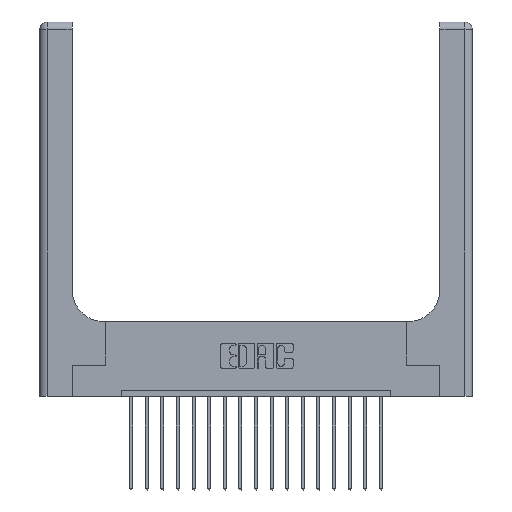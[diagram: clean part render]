
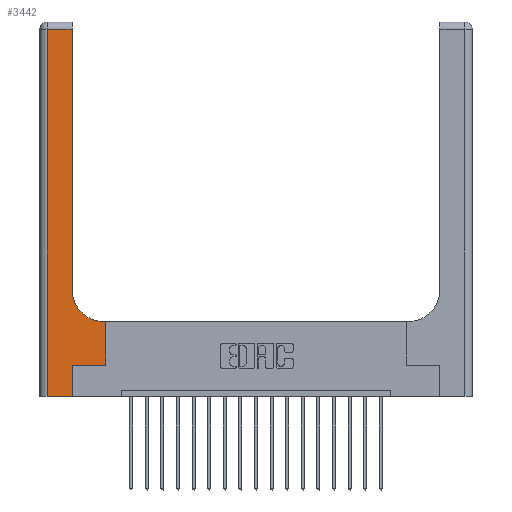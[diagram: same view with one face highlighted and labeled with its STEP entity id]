
A CAD part, top view. The second image highlights one B-rep face of the part: STEP entity #3442.
In plain terms, the highlighted planar face has unit normal (0, 0, 1).
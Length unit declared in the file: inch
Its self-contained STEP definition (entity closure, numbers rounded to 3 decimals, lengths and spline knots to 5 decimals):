
#392 = EDGE_CURVE ( 'NONE', #11306, #8371, #546, .T. ) ;
#546 = LINE ( 'NONE', #15489, #1305 ) ;
#905 = ORIENTED_EDGE ( 'NONE', *, *, #8305, .T. ) ;
#1125 = CARTESIAN_POINT ( 'NONE',  ( 0.528, 0.6, 0.37 ) ) ;
#1305 = VECTOR ( 'NONE', #1927, 39.37008 ) ;
#1346 = VERTEX_POINT ( 'NONE', #19489 ) ;
#1441 = PLANE ( 'NONE',  #3773 ) ;
#1927 = DIRECTION ( 'NONE',  ( -1., 0., 0. ) ) ;
#2110 = VECTOR ( 'NONE', #17994, 39.37008 ) ;
#2595 = VERTEX_POINT ( 'NONE', #19291 ) ;
#2702 = CARTESIAN_POINT ( 'NONE',  ( 0.26, 3., 0.37 ) ) ;
#2957 = DIRECTION ( 'NONE',  ( 1., 0., 0. ) ) ;
#3047 = LINE ( 'NONE', #13448, #5927 ) ;
#3172 = VECTOR ( 'NONE', #16935, 39.37008 ) ;
#3442 = ADVANCED_FACE ( 'NONE', ( #5811 ), #1441, .F. ) ;
#3724 = ORIENTED_EDGE ( 'NONE', *, *, #392, .T. ) ;
#3773 = AXIS2_PLACEMENT_3D ( 'NONE', #11852, #18048, #5622 ) ;
#3838 = DIRECTION ( 'NONE',  ( 1., 0., 0. ) ) ;
#4240 = EDGE_CURVE ( 'NONE', #18303, #2595, #16320, .T. ) ;
#4498 = EDGE_LOOP ( 'NONE', ( #5626, #13024, #5891, #18008, #6142, #13598, #11225, #3724, #905 ) ) ;
#4603 = VERTEX_POINT ( 'NONE', #18040 ) ;
#4831 = EDGE_CURVE ( 'NONE', #1346, #13852, #7162, .T. ) ;
#5211 = CARTESIAN_POINT ( 'NONE',  ( 0.265, 0.25, 0.37 ) ) ;
#5312 = EDGE_CURVE ( 'NONE', #2595, #11306, #7324, .T. ) ;
#5443 = CARTESIAN_POINT ( 'NONE',  ( 0.26, 2.94, 0.37 ) ) ;
#5523 = CARTESIAN_POINT ( 'NONE',  ( 0.51, 0.6, 0.37 ) ) ;
#5589 = DIRECTION ( 'NONE',  ( 0., 1., 0. ) ) ;
#5622 = DIRECTION ( 'NONE',  ( -1., 0., 0. ) ) ;
#5626 = ORIENTED_EDGE ( 'NONE', *, *, #4831, .T. ) ;
#5672 = EDGE_CURVE ( 'NONE', #12460, #9512, #3047, .T. ) ;
#5811 = FACE_OUTER_BOUND ( 'NONE', #4498, .T. ) ;
#5891 = ORIENTED_EDGE ( 'NONE', *, *, #14929, .T. ) ;
#5927 = VECTOR ( 'NONE', #7399, 39.37008 ) ;
#6142 = ORIENTED_EDGE ( 'NONE', *, *, #12704, .T. ) ;
#6262 = CARTESIAN_POINT ( 'NONE',  ( 0.06, 3., 0.37 ) ) ;
#7162 = LINE ( 'NONE', #2702, #17576 ) ;
#7324 = LINE ( 'NONE', #11893, #2110 ) ;
#7399 = DIRECTION ( 'NONE',  ( 1., 0., 0. ) ) ;
#8305 = EDGE_CURVE ( 'NONE', #8371, #1346, #9919, .T. ) ;
#8371 = VERTEX_POINT ( 'NONE', #5523 ) ;
#8415 = VECTOR ( 'NONE', #2957, 39.37008 ) ;
#8953 = LINE ( 'NONE', #13700, #14681 ) ;
#9038 = LINE ( 'NONE', #6262, #3172 ) ;
#9512 = VERTEX_POINT ( 'NONE', #15595 ) ;
#9919 = CIRCLE ( 'NONE', #12448, 0.25 ) ;
#9973 = DIRECTION ( 'NONE',  ( 0., 0., -1. ) ) ;
#10404 = VECTOR ( 'NONE', #13657, 39.37008 ) ;
#11225 = ORIENTED_EDGE ( 'NONE', *, *, #5312, .T. ) ;
#11306 = VERTEX_POINT ( 'NONE', #1125 ) ;
#11370 = CARTESIAN_POINT ( 'NONE',  ( 0.51, 0.85, 0.37 ) ) ;
#11852 = CARTESIAN_POINT ( 'NONE',  ( 0., 3., 0.37 ) ) ;
#11893 = CARTESIAN_POINT ( 'NONE',  ( 0.528, 0.25, 0.37 ) ) ;
#12448 = AXIS2_PLACEMENT_3D ( 'NONE', #11370, #9973, #3838 ) ;
#12460 = VERTEX_POINT ( 'NONE', #18806 ) ;
#12704 = EDGE_CURVE ( 'NONE', #9512, #18303, #15429, .T. ) ;
#13024 = ORIENTED_EDGE ( 'NONE', *, *, #18553, .T. ) ;
#13448 = CARTESIAN_POINT ( 'NONE',  ( 0., 0., 0.37 ) ) ;
#13598 = ORIENTED_EDGE ( 'NONE', *, *, #4240, .T. ) ;
#13657 = DIRECTION ( 'NONE',  ( 0., 1., 0. ) ) ;
#13700 = CARTESIAN_POINT ( 'NONE',  ( 0., 2.94, 0.37 ) ) ;
#13852 = VERTEX_POINT ( 'NONE', #5443 ) ;
#14051 = CARTESIAN_POINT ( 'NONE',  ( 0.265, 0., 0.37 ) ) ;
#14681 = VECTOR ( 'NONE', #15001, 39.37008 ) ;
#14929 = EDGE_CURVE ( 'NONE', #4603, #12460, #9038, .T. ) ;
#15001 = DIRECTION ( 'NONE',  ( -1., 0., 0. ) ) ;
#15429 = LINE ( 'NONE', #14051, #10404 ) ;
#15489 = CARTESIAN_POINT ( 'NONE',  ( 0.26, 0.6, 0.37 ) ) ;
#15595 = CARTESIAN_POINT ( 'NONE',  ( 0.265, 0., 0.37 ) ) ;
#16320 = LINE ( 'NONE', #16409, #8415 ) ;
#16409 = CARTESIAN_POINT ( 'NONE',  ( 0.265, 0.25, 0.37 ) ) ;
#16935 = DIRECTION ( 'NONE',  ( 0., -1., 0. ) ) ;
#17576 = VECTOR ( 'NONE', #5589, 39.37008 ) ;
#17994 = DIRECTION ( 'NONE',  ( 0., 1., 0. ) ) ;
#18008 = ORIENTED_EDGE ( 'NONE', *, *, #5672, .T. ) ;
#18040 = CARTESIAN_POINT ( 'NONE',  ( 0.06, 2.94, 0.37 ) ) ;
#18048 = DIRECTION ( 'NONE',  ( 0., 0., -1. ) ) ;
#18303 = VERTEX_POINT ( 'NONE', #5211 ) ;
#18553 = EDGE_CURVE ( 'NONE', #13852, #4603, #8953, .T. ) ;
#18806 = CARTESIAN_POINT ( 'NONE',  ( 0.06, 0., 0.37 ) ) ;
#19291 = CARTESIAN_POINT ( 'NONE',  ( 0.528, 0.25, 0.37 ) ) ;
#19489 = CARTESIAN_POINT ( 'NONE',  ( 0.26, 0.85, 0.37 ) ) ;
